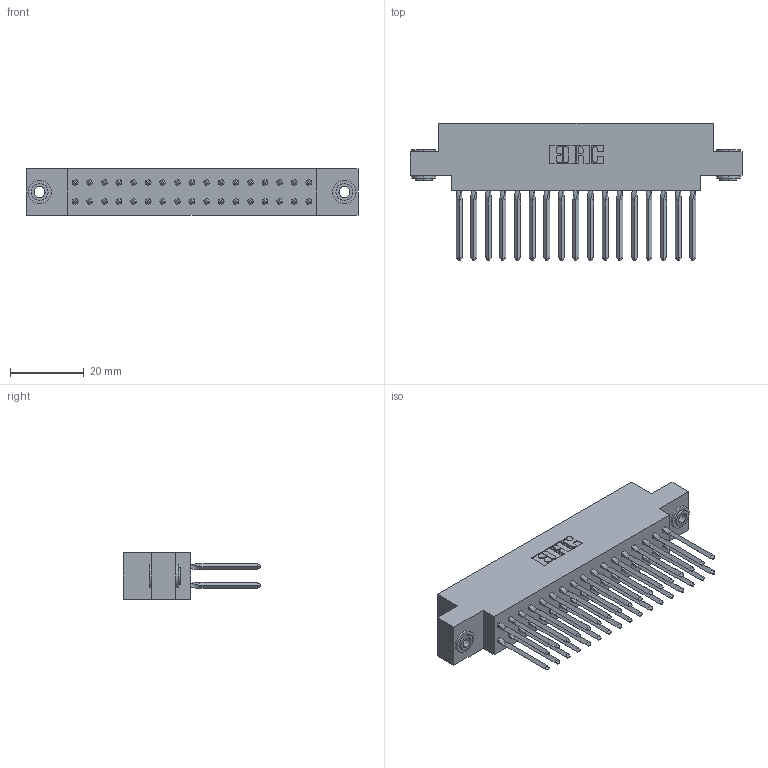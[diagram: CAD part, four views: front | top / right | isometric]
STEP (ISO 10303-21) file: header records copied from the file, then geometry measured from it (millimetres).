
FILE_DESCRIPTION (( 'STEP AP203' ), '1' );
FILE_NAME ('317-034-542-803.STEP', '2020-02-27T22:01:56', ( '' ), ( '' ), 'SwSTEP 2.0', 'SolidWorks 2016', '' );
FILE_SCHEMA (( 'CONFIG_CONTROL_DESIGN' ));
Length unit declared in the file: inch
Products named in the file (4): 345-250-002_345-250-002-102; 317-034-542-803; 317 Part_.156 Dia - TH; 317-290-003_542
Assembly tree (37 placements, depth 2):
  317-034-542-803
    317 Part_.156 Dia - TH
    317-290-003_542  x34
    345-250-002_345-250-002-102  x2
Bounding box: 90.07 x 37.34 x 12.7 mm (x, y, z)
Volume: 13977.7 mm3; surface area: 18851.4 mm2
Topology: 37 solids, 37 shells, 2078 faces, 5791 edges, 3698 vertices
Faces by surface type: plane 1632, cylinder 302, bspline 136, cone 8
Entity records: 27728 total; most frequent: CARTESIAN_POINT 5052, ORIENTED_EDGE 4708, DIRECTION 4044, EDGE_CURVE 2354, LINE 2160, VECTOR 2160, VERTEX_POINT 1562, AXIS2_PLACEMENT_3D 942
